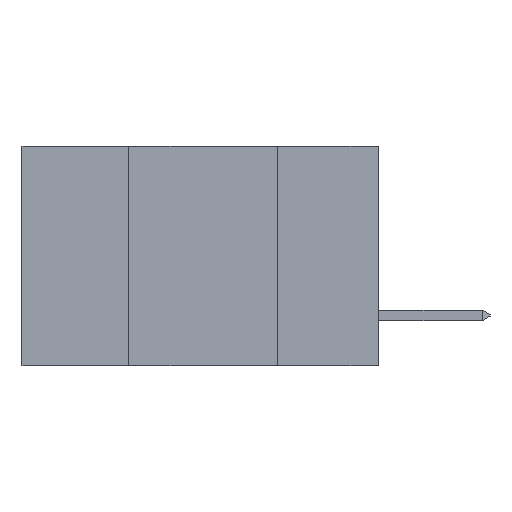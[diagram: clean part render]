
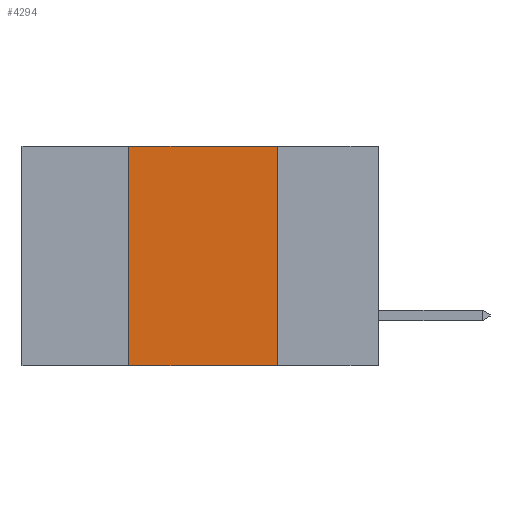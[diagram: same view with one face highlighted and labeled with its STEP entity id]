
A CAD part, left-side view. The second image highlights one B-rep face of the part: STEP entity #4294.
In plain terms, the highlighted planar face has unit normal (-1, 0, 0).
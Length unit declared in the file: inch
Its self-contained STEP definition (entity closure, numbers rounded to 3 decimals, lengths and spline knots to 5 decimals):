
#225 = CARTESIAN_POINT ( 'NONE',  ( 0., 0.6, -0.37 ) ) ;
#419 = ORIENTED_EDGE ( 'NONE', *, *, #2405, .F. ) ;
#521 = ORIENTED_EDGE ( 'NONE', *, *, #5263, .T. ) ;
#680 = DIRECTION ( 'NONE',  ( 0., -1., 0. ) ) ;
#992 = LINE ( 'NONE', #225, #5170 ) ;
#1018 = DIRECTION ( 'NONE',  ( 0., -1., 0. ) ) ;
#1268 = FACE_OUTER_BOUND ( 'NONE', #4997, .T. ) ;
#1669 = ORIENTED_EDGE ( 'NONE', *, *, #2984, .F. ) ;
#1821 = ORIENTED_EDGE ( 'NONE', *, *, #7904, .F. ) ;
#1851 = LINE ( 'NONE', #7060, #6242 ) ;
#2387 = VERTEX_POINT ( 'NONE', #4178 ) ;
#2405 = EDGE_CURVE ( 'NONE', #3535, #6083, #1851, .T. ) ;
#2580 = VERTEX_POINT ( 'NONE', #9568 ) ;
#2921 = AXIS2_PLACEMENT_3D ( 'NONE', #6760, #6706, #6691 ) ;
#2984 = EDGE_CURVE ( 'NONE', #2580, #3535, #3882, .T. ) ;
#3535 = VERTEX_POINT ( 'NONE', #7670 ) ;
#3882 = LINE ( 'NONE', #7761, #9619 ) ;
#4178 = CARTESIAN_POINT ( 'NONE',  ( 0., 0.17, -0.37 ) ) ;
#4294 = ADVANCED_FACE ( 'NONE', ( #1268 ), #6725, .F. ) ;
#4997 = EDGE_LOOP ( 'NONE', ( #1821, #419, #1669, #521 ) ) ;
#5170 = VECTOR ( 'NONE', #1018, 39.37008 ) ;
#5263 = EDGE_CURVE ( 'NONE', #2580, #2387, #992, .T. ) ;
#6083 = VERTEX_POINT ( 'NONE', #6607 ) ;
#6242 = VECTOR ( 'NONE', #680, 39.37008 ) ;
#6607 = CARTESIAN_POINT ( 'NONE',  ( 0., 0.17, 0. ) ) ;
#6647 = VECTOR ( 'NONE', #9357, 39.37008 ) ;
#6691 = DIRECTION ( 'NONE',  ( 0., 0., -1. ) ) ;
#6706 = DIRECTION ( 'NONE',  ( 1., 0., 0. ) ) ;
#6725 = PLANE ( 'NONE',  #2921 ) ;
#6760 = CARTESIAN_POINT ( 'NONE',  ( 0., 0.6, 0. ) ) ;
#7060 = CARTESIAN_POINT ( 'NONE',  ( 0., 0.6, 0. ) ) ;
#7189 = CARTESIAN_POINT ( 'NONE',  ( 0., 0.17, -0.37 ) ) ;
#7670 = CARTESIAN_POINT ( 'NONE',  ( 0., 0.42, 0. ) ) ;
#7761 = CARTESIAN_POINT ( 'NONE',  ( 0., 0.42, -0.37 ) ) ;
#7904 = EDGE_CURVE ( 'NONE', #6083, #2387, #8573, .T. ) ;
#8573 = LINE ( 'NONE', #7189, #6647 ) ;
#9194 = DIRECTION ( 'NONE',  ( 0., 0., 1. ) ) ;
#9357 = DIRECTION ( 'NONE',  ( 0., 0., -1. ) ) ;
#9568 = CARTESIAN_POINT ( 'NONE',  ( 0., 0.42, -0.37 ) ) ;
#9619 = VECTOR ( 'NONE', #9194, 39.37008 ) ;
